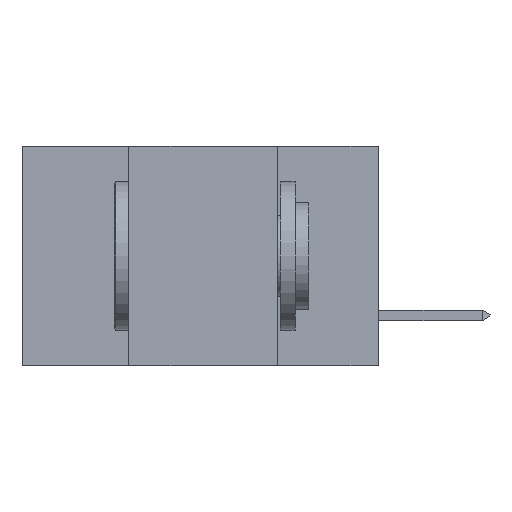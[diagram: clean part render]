
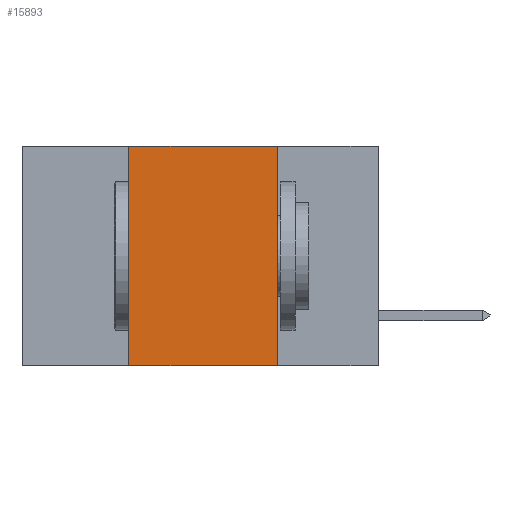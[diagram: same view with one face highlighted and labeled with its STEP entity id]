
A CAD part, left-side view. The second image highlights one B-rep face of the part: STEP entity #15893.
In plain terms, the highlighted planar face has unit normal (-1, 0, 0).
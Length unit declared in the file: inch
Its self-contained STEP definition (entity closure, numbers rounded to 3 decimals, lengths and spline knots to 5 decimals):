
#554 = VERTEX_POINT ( 'NONE', #8616 ) ;
#1516 = EDGE_CURVE ( 'NONE', #554, #9039, #13594, .T. ) ;
#1920 = CARTESIAN_POINT ( 'NONE',  ( 0., 0.6, -0.37 ) ) ;
#1921 = VECTOR ( 'NONE', #3331, 39.37008 ) ;
#2307 = ORIENTED_EDGE ( 'NONE', *, *, #1516, .F. ) ;
#3331 = DIRECTION ( 'NONE',  ( 0., 0., 1. ) ) ;
#3423 = EDGE_LOOP ( 'NONE', ( #3650, #2307, #14140, #4876 ) ) ;
#3650 = ORIENTED_EDGE ( 'NONE', *, *, #10759, .F. ) ;
#4437 = VECTOR ( 'NONE', #8004, 39.37008 ) ;
#4876 = ORIENTED_EDGE ( 'NONE', *, *, #17422, .T. ) ;
#5519 = CARTESIAN_POINT ( 'NONE',  ( 0., 0.6, 0. ) ) ;
#6904 = FACE_OUTER_BOUND ( 'NONE', #3423, .T. ) ;
#7025 = AXIS2_PLACEMENT_3D ( 'NONE', #5519, #13721, #17984 ) ;
#7343 = DIRECTION ( 'NONE',  ( 0., 0., -1. ) ) ;
#7739 = LINE ( 'NONE', #1920, #15444 ) ;
#8004 = DIRECTION ( 'NONE',  ( 0., -1., 0. ) ) ;
#8616 = CARTESIAN_POINT ( 'NONE',  ( 0., 0.42, 0. ) ) ;
#8709 = VERTEX_POINT ( 'NONE', #14639 ) ;
#8890 = VECTOR ( 'NONE', #7343, 39.37008 ) ;
#9039 = VERTEX_POINT ( 'NONE', #16791 ) ;
#10698 = LINE ( 'NONE', #16385, #1921 ) ;
#10759 = EDGE_CURVE ( 'NONE', #9039, #11728, #17128, .T. ) ;
#11728 = VERTEX_POINT ( 'NONE', #15610 ) ;
#12011 = DIRECTION ( 'NONE',  ( 0., -1., 0. ) ) ;
#12601 = PLANE ( 'NONE',  #7025 ) ;
#13320 = CARTESIAN_POINT ( 'NONE',  ( 0., 0.6, 0. ) ) ;
#13594 = LINE ( 'NONE', #13320, #4437 ) ;
#13721 = DIRECTION ( 'NONE',  ( 1., 0., 0. ) ) ;
#14140 = ORIENTED_EDGE ( 'NONE', *, *, #15337, .F. ) ;
#14261 = CARTESIAN_POINT ( 'NONE',  ( 0., 0.17, -0.37 ) ) ;
#14639 = CARTESIAN_POINT ( 'NONE',  ( 0., 0.42, -0.37 ) ) ;
#15337 = EDGE_CURVE ( 'NONE', #8709, #554, #10698, .T. ) ;
#15444 = VECTOR ( 'NONE', #12011, 39.37008 ) ;
#15610 = CARTESIAN_POINT ( 'NONE',  ( 0., 0.17, -0.37 ) ) ;
#15893 = ADVANCED_FACE ( 'NONE', ( #6904 ), #12601, .F. ) ;
#16385 = CARTESIAN_POINT ( 'NONE',  ( 0., 0.42, -0.37 ) ) ;
#16791 = CARTESIAN_POINT ( 'NONE',  ( 0., 0.17, 0. ) ) ;
#17128 = LINE ( 'NONE', #14261, #8890 ) ;
#17422 = EDGE_CURVE ( 'NONE', #8709, #11728, #7739, .T. ) ;
#17984 = DIRECTION ( 'NONE',  ( 0., 0., -1. ) ) ;
